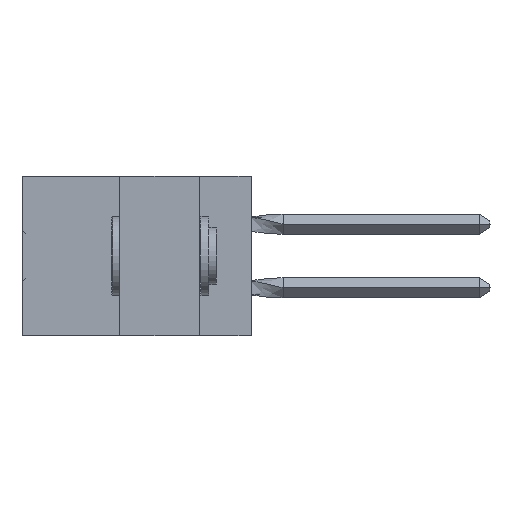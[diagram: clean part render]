
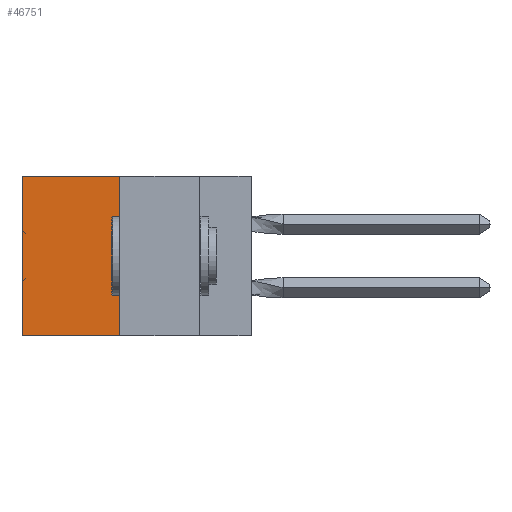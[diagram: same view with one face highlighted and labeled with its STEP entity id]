
A CAD part, left-side view. The second image highlights one B-rep face of the part: STEP entity #46751.
In plain terms, the highlighted planar face has unit normal (-1, 0, 0).
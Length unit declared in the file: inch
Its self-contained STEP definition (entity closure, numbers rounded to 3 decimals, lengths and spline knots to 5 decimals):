
#507 = EDGE_CURVE ( 'NONE', #23834, #5343, #28966, .T. ) ;
#1066 = VERTEX_POINT ( 'NONE', #27098 ) ;
#1597 = CARTESIAN_POINT ( 'NONE',  ( 0.305, 0.413, -0.5 ) ) ;
#2572 = DIRECTION ( 'NONE',  ( 1., 0., 0. ) ) ;
#5343 = VERTEX_POINT ( 'NONE', #50570 ) ;
#5586 = DIRECTION ( 'NONE',  ( 0., 0., -1. ) ) ;
#9412 = EDGE_CURVE ( 'NONE', #27199, #23834, #31208, .T. ) ;
#9931 = VECTOR ( 'NONE', #50523, 39.37008 ) ;
#14997 = CARTESIAN_POINT ( 'NONE',  ( 0.305, 0.413, -0.5 ) ) ;
#19645 = EDGE_CURVE ( 'NONE', #1066, #5343, #54409, .T. ) ;
#22668 = CARTESIAN_POINT ( 'NONE',  ( 0.305, 0.413, -0.5 ) ) ;
#23613 = VECTOR ( 'NONE', #31777, 39.37008 ) ;
#23834 = VERTEX_POINT ( 'NONE', #1597 ) ;
#24121 = CARTESIAN_POINT ( 'NONE',  ( 0.305, 0.413, 0. ) ) ;
#24265 = DIRECTION ( 'NONE',  ( 0., 0., -1. ) ) ;
#24407 = VECTOR ( 'NONE', #36943, 39.37008 ) ;
#24720 = ORIENTED_EDGE ( 'NONE', *, *, #19645, .T. ) ;
#27098 = CARTESIAN_POINT ( 'NONE',  ( 0.305, 0.72, 0. ) ) ;
#27199 = VERTEX_POINT ( 'NONE', #48973 ) ;
#27549 = ORIENTED_EDGE ( 'NONE', *, *, #9412, .F. ) ;
#28966 = LINE ( 'NONE', #22668, #23613 ) ;
#29491 = FACE_OUTER_BOUND ( 'NONE', #47496, .T. ) ;
#30466 = EDGE_CURVE ( 'NONE', #27199, #1066, #35716, .T. ) ;
#31208 = LINE ( 'NONE', #33523, #9931 ) ;
#31777 = DIRECTION ( 'NONE',  ( 0., 1., 0. ) ) ;
#32422 = VECTOR ( 'NONE', #5586, 39.37008 ) ;
#33523 = CARTESIAN_POINT ( 'NONE',  ( 0.305, 0.413, -0.5 ) ) ;
#35716 = LINE ( 'NONE', #24121, #24407 ) ;
#36943 = DIRECTION ( 'NONE',  ( 0., 1., 0. ) ) ;
#40672 = PLANE ( 'NONE',  #46599 ) ;
#41490 = ORIENTED_EDGE ( 'NONE', *, *, #507, .F. ) ;
#46599 = AXIS2_PLACEMENT_3D ( 'NONE', #14997, #2572, #24265 ) ;
#46751 = ADVANCED_FACE ( 'NONE', ( #29491 ), #40672, .F. ) ;
#47496 = EDGE_LOOP ( 'NONE', ( #24720, #41490, #27549, #48265 ) ) ;
#48265 = ORIENTED_EDGE ( 'NONE', *, *, #30466, .T. ) ;
#48973 = CARTESIAN_POINT ( 'NONE',  ( 0.305, 0.413, 0. ) ) ;
#50523 = DIRECTION ( 'NONE',  ( 0., 0., -1. ) ) ;
#50570 = CARTESIAN_POINT ( 'NONE',  ( 0.305, 0.72, -0.5 ) ) ;
#51774 = CARTESIAN_POINT ( 'NONE',  ( 0.305, 0.72, -0.5 ) ) ;
#54409 = LINE ( 'NONE', #51774, #32422 ) ;
